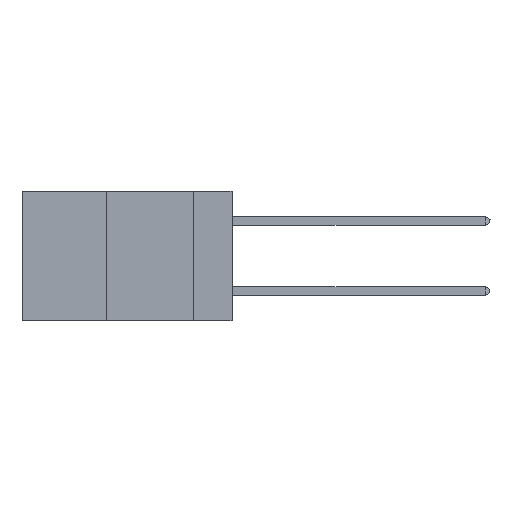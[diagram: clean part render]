
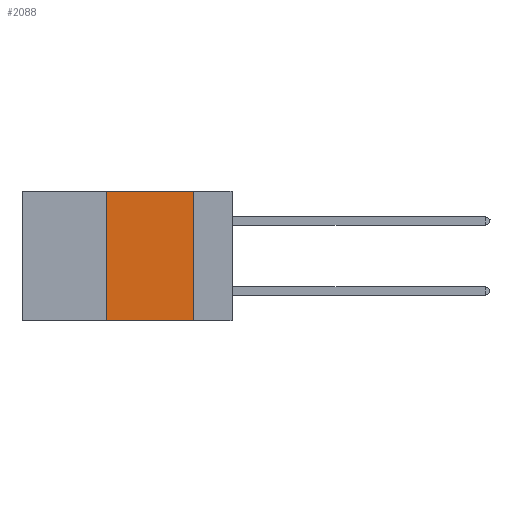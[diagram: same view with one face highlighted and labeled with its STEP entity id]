
A CAD part, left-side view. The second image highlights one B-rep face of the part: STEP entity #2088.
In plain terms, the highlighted planar face has unit normal (-1, 0, 0).
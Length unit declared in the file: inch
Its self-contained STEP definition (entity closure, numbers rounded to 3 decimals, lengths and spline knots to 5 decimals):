
#585 = VECTOR ( 'NONE', #10434, 39.37008 ) ;
#1072 = DIRECTION ( 'NONE',  ( 0., -1., 0. ) ) ;
#1571 = VERTEX_POINT ( 'NONE', #10934 ) ;
#1695 = CARTESIAN_POINT ( 'NONE',  ( 0., 0.36, 0. ) ) ;
#2054 = ORIENTED_EDGE ( 'NONE', *, *, #3912, .T. ) ;
#2088 = ADVANCED_FACE ( 'NONE', ( #15633 ), #11586, .F. ) ;
#2697 = CARTESIAN_POINT ( 'NONE',  ( 0., 0.6, -0.37 ) ) ;
#3858 = EDGE_LOOP ( 'NONE', ( #5641, #11106, #7375, #2054 ) ) ;
#3912 = EDGE_CURVE ( 'NONE', #5042, #18820, #9817, .T. ) ;
#5042 = VERTEX_POINT ( 'NONE', #6380 ) ;
#5641 = ORIENTED_EDGE ( 'NONE', *, *, #14353, .F. ) ;
#6241 = EDGE_CURVE ( 'NONE', #5042, #15087, #11878, .T. ) ;
#6380 = CARTESIAN_POINT ( 'NONE',  ( 0., 0.36, -0.37 ) ) ;
#7375 = ORIENTED_EDGE ( 'NONE', *, *, #6241, .F. ) ;
#7926 = LINE ( 'NONE', #13556, #10898 ) ;
#9817 = LINE ( 'NONE', #2697, #17192 ) ;
#9838 = CARTESIAN_POINT ( 'NONE',  ( 0., 0.11, -0.37 ) ) ;
#9886 = VECTOR ( 'NONE', #13019, 39.37008 ) ;
#10434 = DIRECTION ( 'NONE',  ( 0., 0., 1. ) ) ;
#10898 = VECTOR ( 'NONE', #15274, 39.37008 ) ;
#10934 = CARTESIAN_POINT ( 'NONE',  ( 0., 0.11, 0. ) ) ;
#11083 = EDGE_CURVE ( 'NONE', #15087, #1571, #18804, .T. ) ;
#11106 = ORIENTED_EDGE ( 'NONE', *, *, #11083, .F. ) ;
#11486 = DIRECTION ( 'NONE',  ( 1., 0., 0. ) ) ;
#11586 = PLANE ( 'NONE',  #16501 ) ;
#11878 = LINE ( 'NONE', #13527, #585 ) ;
#13019 = DIRECTION ( 'NONE',  ( 0., -1., 0. ) ) ;
#13527 = CARTESIAN_POINT ( 'NONE',  ( 0., 0.36, 0. ) ) ;
#13556 = CARTESIAN_POINT ( 'NONE',  ( 0., 0.11, 0. ) ) ;
#14353 = EDGE_CURVE ( 'NONE', #1571, #18820, #7926, .T. ) ;
#15087 = VERTEX_POINT ( 'NONE', #1695 ) ;
#15274 = DIRECTION ( 'NONE',  ( 0., 0., -1. ) ) ;
#15633 = FACE_OUTER_BOUND ( 'NONE', #3858, .T. ) ;
#16198 = CARTESIAN_POINT ( 'NONE',  ( 0., 0.6, 0. ) ) ;
#16501 = AXIS2_PLACEMENT_3D ( 'NONE', #17083, #11486, #18515 ) ;
#17083 = CARTESIAN_POINT ( 'NONE',  ( 0., 0.6, 0. ) ) ;
#17192 = VECTOR ( 'NONE', #1072, 39.37008 ) ;
#18515 = DIRECTION ( 'NONE',  ( 0., 0., -1. ) ) ;
#18804 = LINE ( 'NONE', #16198, #9886 ) ;
#18820 = VERTEX_POINT ( 'NONE', #9838 ) ;
